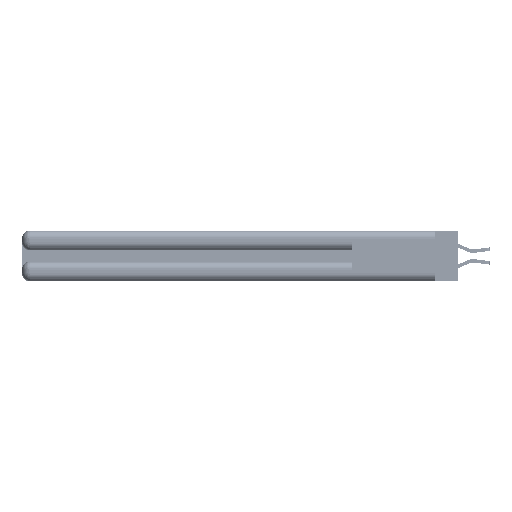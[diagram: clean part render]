
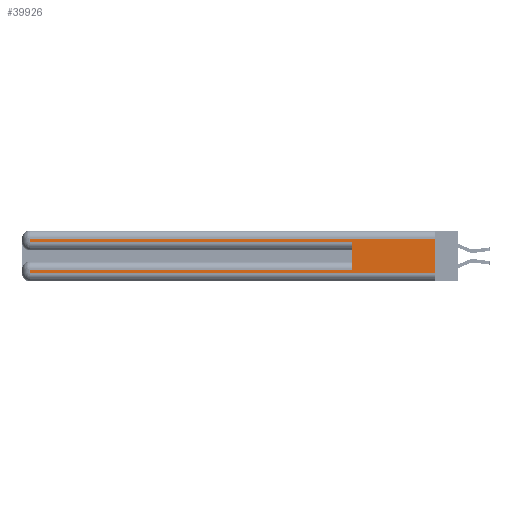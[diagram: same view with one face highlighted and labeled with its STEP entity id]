
A CAD part, left-side view. The second image highlights one B-rep face of the part: STEP entity #39926.
In plain terms, the highlighted planar face has unit normal (-1, 0, 0).
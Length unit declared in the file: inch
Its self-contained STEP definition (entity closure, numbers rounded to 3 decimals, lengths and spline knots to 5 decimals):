
#309 = CARTESIAN_POINT ( 'NONE',  ( 0., 0.6, 0.085 ) ) ;
#401 = ORIENTED_EDGE ( 'NONE', *, *, #41140, .T. ) ;
#609 = VERTEX_POINT ( 'NONE', #19227 ) ;
#717 = CARTESIAN_POINT ( 'NONE',  ( 0., 2.94, 0.31 ) ) ;
#842 = DIRECTION ( 'NONE',  ( 0., -1., 0. ) ) ;
#2201 = VECTOR ( 'NONE', #35240, 39.37008 ) ;
#2474 = CARTESIAN_POINT ( 'NONE',  ( 0., 2.94, 0.085 ) ) ;
#2498 = DIRECTION ( 'NONE',  ( 0., 0., 1. ) ) ;
#3573 = CARTESIAN_POINT ( 'NONE',  ( 0., 0., 0.06 ) ) ;
#3904 = LINE ( 'NONE', #41581, #4999 ) ;
#4999 = VECTOR ( 'NONE', #24549, 39.37008 ) ;
#6166 = VERTEX_POINT ( 'NONE', #2474 ) ;
#6331 = ORIENTED_EDGE ( 'NONE', *, *, #23263, .T. ) ;
#7043 = VERTEX_POINT ( 'NONE', #717 ) ;
#7714 = ORIENTED_EDGE ( 'NONE', *, *, #9917, .T. ) ;
#7801 = LINE ( 'NONE', #31815, #43139 ) ;
#9764 = DIRECTION ( 'NONE',  ( 0., 1., 0. ) ) ;
#9917 = EDGE_CURVE ( 'NONE', #609, #38824, #30114, .T. ) ;
#10057 = DIRECTION ( 'NONE',  ( 0., 0., -1. ) ) ;
#11249 = DIRECTION ( 'NONE',  ( 0., -1., 0. ) ) ;
#11349 = CARTESIAN_POINT ( 'NONE',  ( 0., 0., 0.285 ) ) ;
#11843 = VECTOR ( 'NONE', #842, 39.37008 ) ;
#12272 = EDGE_LOOP ( 'NONE', ( #30392, #6331, #33722, #7714, #40817, #31150, #401, #23858 ) ) ;
#12869 = LINE ( 'NONE', #26610, #30040 ) ;
#13315 = EDGE_CURVE ( 'NONE', #7043, #609, #20575, .T. ) ;
#14418 = EDGE_CURVE ( 'NONE', #14753, #6166, #40287, .T. ) ;
#14753 = VERTEX_POINT ( 'NONE', #309 ) ;
#14824 = CARTESIAN_POINT ( 'NONE',  ( 0., 2.94, 0.06 ) ) ;
#15204 = CARTESIAN_POINT ( 'NONE',  ( 0., 0., 0.085 ) ) ;
#15469 = CARTESIAN_POINT ( 'NONE',  ( 0., 0.6, 0.285 ) ) ;
#15937 = FACE_OUTER_BOUND ( 'NONE', #12272, .T. ) ;
#19227 = CARTESIAN_POINT ( 'NONE',  ( 0., 2.94, 0.285 ) ) ;
#19426 = DIRECTION ( 'NONE',  ( 1., 0., 0. ) ) ;
#20575 = LINE ( 'NONE', #31779, #2201 ) ;
#21391 = AXIS2_PLACEMENT_3D ( 'NONE', #39909, #19426, #43277 ) ;
#23263 = EDGE_CURVE ( 'NONE', #36664, #7043, #35136, .T. ) ;
#23858 = ORIENTED_EDGE ( 'NONE', *, *, #40379, .T. ) ;
#24549 = DIRECTION ( 'NONE',  ( 0., 0., -1. ) ) ;
#25284 = VECTOR ( 'NONE', #39181, 39.37008 ) ;
#25544 = VECTOR ( 'NONE', #10057, 39.37008 ) ;
#25997 = VECTOR ( 'NONE', #9764, 39.37008 ) ;
#26610 = CARTESIAN_POINT ( 'NONE',  ( 0., 0.6, 0.145 ) ) ;
#26626 = LINE ( 'NONE', #40789, #25544 ) ;
#26809 = VERTEX_POINT ( 'NONE', #3573 ) ;
#30040 = VECTOR ( 'NONE', #2498, 39.37008 ) ;
#30114 = LINE ( 'NONE', #11349, #11843 ) ;
#30392 = ORIENTED_EDGE ( 'NONE', *, *, #40118, .F. ) ;
#30500 = VERTEX_POINT ( 'NONE', #14824 ) ;
#31150 = ORIENTED_EDGE ( 'NONE', *, *, #14418, .T. ) ;
#31779 = CARTESIAN_POINT ( 'NONE',  ( 0., 2.94, 0.37 ) ) ;
#31815 = CARTESIAN_POINT ( 'NONE',  ( 0., 0., 0.06 ) ) ;
#33044 = PLANE ( 'NONE',  #21391 ) ;
#33638 = CARTESIAN_POINT ( 'NONE',  ( 0., 0., 0.31 ) ) ;
#33722 = ORIENTED_EDGE ( 'NONE', *, *, #13315, .T. ) ;
#34450 = EDGE_CURVE ( 'NONE', #14753, #38824, #12869, .T. ) ;
#35136 = LINE ( 'NONE', #33638, #25997 ) ;
#35240 = DIRECTION ( 'NONE',  ( 0., 0., -1. ) ) ;
#36664 = VERTEX_POINT ( 'NONE', #36970 ) ;
#36970 = CARTESIAN_POINT ( 'NONE',  ( 0., 0., 0.31 ) ) ;
#38824 = VERTEX_POINT ( 'NONE', #15469 ) ;
#39181 = DIRECTION ( 'NONE',  ( 0., 1., 0. ) ) ;
#39909 = CARTESIAN_POINT ( 'NONE',  ( 0., 0., 0.37 ) ) ;
#39926 = ADVANCED_FACE ( 'NONE', ( #15937 ), #33044, .F. ) ;
#40118 = EDGE_CURVE ( 'NONE', #36664, #26809, #26626, .T. ) ;
#40287 = LINE ( 'NONE', #15204, #25284 ) ;
#40379 = EDGE_CURVE ( 'NONE', #30500, #26809, #7801, .T. ) ;
#40789 = CARTESIAN_POINT ( 'NONE',  ( 0., 0., 0.37 ) ) ;
#40817 = ORIENTED_EDGE ( 'NONE', *, *, #34450, .F. ) ;
#41140 = EDGE_CURVE ( 'NONE', #6166, #30500, #3904, .T. ) ;
#41581 = CARTESIAN_POINT ( 'NONE',  ( 0., 2.94, 0.37 ) ) ;
#43139 = VECTOR ( 'NONE', #11249, 39.37008 ) ;
#43277 = DIRECTION ( 'NONE',  ( 0., 0., -1. ) ) ;
